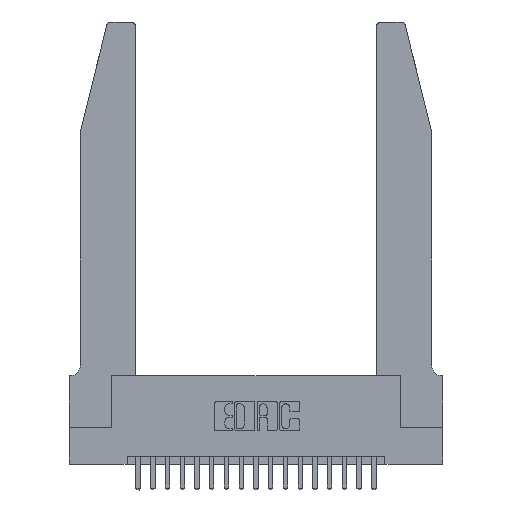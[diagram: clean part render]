
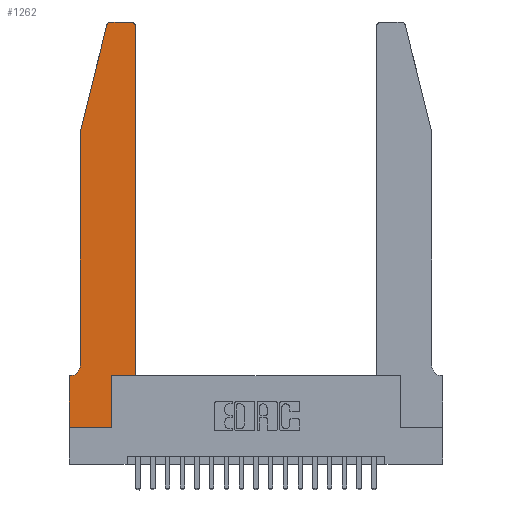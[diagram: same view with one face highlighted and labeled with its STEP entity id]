
A CAD part, top view. The second image highlights one B-rep face of the part: STEP entity #1262.
In plain terms, the highlighted planar face has unit normal (0, 0, 1).
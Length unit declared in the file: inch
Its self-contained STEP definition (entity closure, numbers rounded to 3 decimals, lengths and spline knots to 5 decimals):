
#97 = VECTOR ( 'NONE', #1366, 39.37008 ) ;
#114 = CARTESIAN_POINT ( 'NONE',  ( 0.0755, 0.35, 0.37 ) ) ;
#268 = EDGE_CURVE ( 'NONE', #4019, #9549, #16995, .T. ) ;
#296 = CARTESIAN_POINT ( 'NONE',  ( 0.4505, 0.35, 0.37 ) ) ;
#772 = DIRECTION ( 'NONE',  ( 1., 0., 0. ) ) ;
#1104 = DIRECTION ( 'NONE',  ( 1., 0., 0. ) ) ;
#1262 = ADVANCED_FACE ( 'NONE', ( #5025 ), #7557, .T. ) ;
#1366 = DIRECTION ( 'NONE',  ( -1., 0., 0. ) ) ;
#1574 = EDGE_CURVE ( 'NONE', #17357, #8369, #15481, .T. ) ;
#1706 = CARTESIAN_POINT ( 'NONE',  ( 0.0755, 2., 0.37 ) ) ;
#2188 = CIRCLE ( 'NONE', #11051, 0.07 ) ;
#2231 = LINE ( 'NONE', #13550, #12151 ) ;
#2331 = CARTESIAN_POINT ( 'NONE',  ( 0.0755, 2., 0.37 ) ) ;
#2395 = CARTESIAN_POINT ( 'NONE',  ( 0.4505, 0.35, 0.37 ) ) ;
#2700 = AXIS2_PLACEMENT_3D ( 'NONE', #7418, #20773, #772 ) ;
#2931 = ORIENTED_EDGE ( 'NONE', *, *, #268, .T. ) ;
#3314 = CARTESIAN_POINT ( 'NONE',  ( 0.2865, 0., 0.37 ) ) ;
#3662 = VERTEX_POINT ( 'NONE', #17779 ) ;
#3807 = VERTEX_POINT ( 'NONE', #11806 ) ;
#3890 = DIRECTION ( 'NONE',  ( 0., 0., 1. ) ) ;
#4019 = VERTEX_POINT ( 'NONE', #2395 ) ;
#4150 = LINE ( 'NONE', #7075, #11966 ) ;
#4151 = VECTOR ( 'NONE', #18698, 39.37008 ) ;
#4241 = CARTESIAN_POINT ( 'NONE',  ( 0.0055, 0.35, 0.37 ) ) ;
#4699 = EDGE_CURVE ( 'NONE', #9549, #3807, #5384, .T. ) ;
#4862 = CARTESIAN_POINT ( 'NONE',  ( 0.4505, 0.35, 0.37 ) ) ;
#5025 = FACE_OUTER_BOUND ( 'NONE', #13187, .T. ) ;
#5384 = CIRCLE ( 'NONE', #16263, 0.03 ) ;
#5475 = CARTESIAN_POINT ( 'NONE',  ( 0.284, 2.75, 0.37 ) ) ;
#5497 = EDGE_CURVE ( 'NONE', #6680, #13643, #15307, .T. ) ;
#5772 = CARTESIAN_POINT ( 'NONE',  ( 0.0055, 0.42, 0.37 ) ) ;
#6471 = VERTEX_POINT ( 'NONE', #4241 ) ;
#6680 = VERTEX_POINT ( 'NONE', #5475 ) ;
#6719 = EDGE_CURVE ( 'NONE', #14380, #6471, #2188, .T. ) ;
#6752 = DIRECTION ( 'NONE',  ( 1., 0., 0. ) ) ;
#7075 = CARTESIAN_POINT ( 'NONE',  ( 0.2865, 0.35, 0.37 ) ) ;
#7145 = ORIENTED_EDGE ( 'NONE', *, *, #20625, .T. ) ;
#7223 = ORIENTED_EDGE ( 'NONE', *, *, #9804, .T. ) ;
#7418 = CARTESIAN_POINT ( 'NONE',  ( 0., 0.35, 0.37 ) ) ;
#7480 = DIRECTION ( 'NONE',  ( 0., 0., -1. ) ) ;
#7557 = PLANE ( 'NONE',  #2700 ) ;
#8147 = EDGE_CURVE ( 'NONE', #6471, #11413, #18463, .T. ) ;
#8369 = VERTEX_POINT ( 'NONE', #3314 ) ;
#8517 = VECTOR ( 'NONE', #11404, 39.37008 ) ;
#8667 = VECTOR ( 'NONE', #12622, 39.37008 ) ;
#9293 = VECTOR ( 'NONE', #20792, 39.37008 ) ;
#9549 = VERTEX_POINT ( 'NONE', #14948 ) ;
#9720 = ORIENTED_EDGE ( 'NONE', *, *, #1574, .T. ) ;
#9804 = EDGE_CURVE ( 'NONE', #3807, #6680, #15746, .T. ) ;
#10598 = CARTESIAN_POINT ( 'NONE',  ( 0.25487, 2.72718, 0.37 ) ) ;
#10702 = VERTEX_POINT ( 'NONE', #2331 ) ;
#10890 = CARTESIAN_POINT ( 'NONE',  ( 0.0755, 2., 0.37 ) ) ;
#11043 = ORIENTED_EDGE ( 'NONE', *, *, #6719, .T. ) ;
#11051 = AXIS2_PLACEMENT_3D ( 'NONE', #5772, #7480, #20897 ) ;
#11257 = ORIENTED_EDGE ( 'NONE', *, *, #20866, .T. ) ;
#11404 = DIRECTION ( 'NONE',  ( -0.239, -0.971, 0. ) ) ;
#11413 = VERTEX_POINT ( 'NONE', #21017 ) ;
#11651 = DIRECTION ( 'NONE',  ( 0., -1., 0. ) ) ;
#11806 = CARTESIAN_POINT ( 'NONE',  ( 0.4205, 2.75, 0.37 ) ) ;
#11852 = EDGE_CURVE ( 'NONE', #8369, #3662, #4150, .T. ) ;
#11966 = VECTOR ( 'NONE', #12250, 39.37008 ) ;
#12065 = ORIENTED_EDGE ( 'NONE', *, *, #5497, .T. ) ;
#12139 = ORIENTED_EDGE ( 'NONE', *, *, #17952, .T. ) ;
#12151 = VECTOR ( 'NONE', #11651, 39.37008 ) ;
#12250 = DIRECTION ( 'NONE',  ( 0., 1., 0. ) ) ;
#12622 = DIRECTION ( 'NONE',  ( 1., 0., 0. ) ) ;
#12941 = LINE ( 'NONE', #1706, #8517 ) ;
#13127 = ORIENTED_EDGE ( 'NONE', *, *, #8147, .T. ) ;
#13187 = EDGE_LOOP ( 'NONE', ( #7223, #12065, #16882, #11257, #11043, #13127, #7145, #9720, #18216, #12139, #2931, #15587 ) ) ;
#13396 = DIRECTION ( 'NONE',  ( 0., 0., 1. ) ) ;
#13466 = CARTESIAN_POINT ( 'NONE',  ( 0.284, 2.72, 0.37 ) ) ;
#13550 = CARTESIAN_POINT ( 'NONE',  ( 0., 0., 0.37 ) ) ;
#13643 = VERTEX_POINT ( 'NONE', #10598 ) ;
#14000 = VECTOR ( 'NONE', #16970, 39.37008 ) ;
#14380 = VERTEX_POINT ( 'NONE', #14558 ) ;
#14558 = CARTESIAN_POINT ( 'NONE',  ( 0.0755, 0.42, 0.37 ) ) ;
#14674 = CARTESIAN_POINT ( 'NONE',  ( 0.2605, 2.75, 0.37 ) ) ;
#14825 = LINE ( 'NONE', #10890, #9293 ) ;
#14948 = CARTESIAN_POINT ( 'NONE',  ( 0.4505, 2.72, 0.37 ) ) ;
#15120 = CARTESIAN_POINT ( 'NONE',  ( 0., 0., 0.37 ) ) ;
#15168 = LINE ( 'NONE', #4862, #19083 ) ;
#15307 = CIRCLE ( 'NONE', #19921, 0.03 ) ;
#15481 = LINE ( 'NONE', #19004, #8667 ) ;
#15587 = ORIENTED_EDGE ( 'NONE', *, *, #4699, .T. ) ;
#15746 = LINE ( 'NONE', #14674, #97 ) ;
#16263 = AXIS2_PLACEMENT_3D ( 'NONE', #18804, #3890, #1104 ) ;
#16722 = DIRECTION ( 'NONE',  ( 1., 0., 0. ) ) ;
#16882 = ORIENTED_EDGE ( 'NONE', *, *, #21149, .T. ) ;
#16970 = DIRECTION ( 'NONE',  ( -1., 0., 0. ) ) ;
#16995 = LINE ( 'NONE', #296, #4151 ) ;
#17357 = VERTEX_POINT ( 'NONE', #15120 ) ;
#17779 = CARTESIAN_POINT ( 'NONE',  ( 0.2865, 0.35, 0.37 ) ) ;
#17952 = EDGE_CURVE ( 'NONE', #3662, #4019, #15168, .T. ) ;
#18216 = ORIENTED_EDGE ( 'NONE', *, *, #11852, .T. ) ;
#18463 = LINE ( 'NONE', #114, #14000 ) ;
#18698 = DIRECTION ( 'NONE',  ( 0., 1., 0. ) ) ;
#18804 = CARTESIAN_POINT ( 'NONE',  ( 0.4205, 2.72, 0.37 ) ) ;
#19004 = CARTESIAN_POINT ( 'NONE',  ( 0., 0., 0.37 ) ) ;
#19083 = VECTOR ( 'NONE', #16722, 39.37008 ) ;
#19921 = AXIS2_PLACEMENT_3D ( 'NONE', #13466, #13396, #6752 ) ;
#20625 = EDGE_CURVE ( 'NONE', #11413, #17357, #2231, .T. ) ;
#20773 = DIRECTION ( 'NONE',  ( 0., 0., 1. ) ) ;
#20792 = DIRECTION ( 'NONE',  ( 0., -1., 0. ) ) ;
#20866 = EDGE_CURVE ( 'NONE', #10702, #14380, #14825, .T. ) ;
#20897 = DIRECTION ( 'NONE',  ( -1., 0., 0. ) ) ;
#21017 = CARTESIAN_POINT ( 'NONE',  ( 0., 0.35, 0.37 ) ) ;
#21149 = EDGE_CURVE ( 'NONE', #13643, #10702, #12941, .T. ) ;
